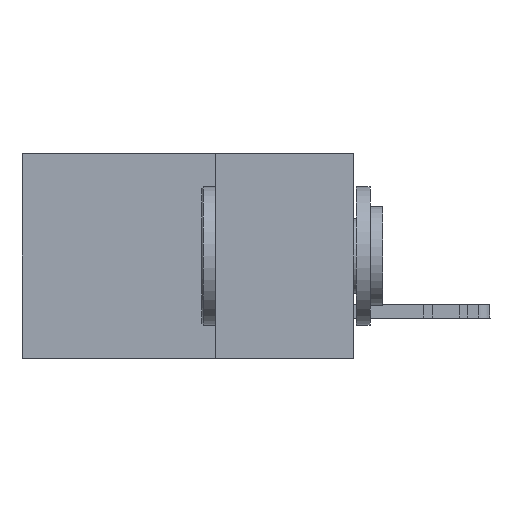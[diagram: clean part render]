
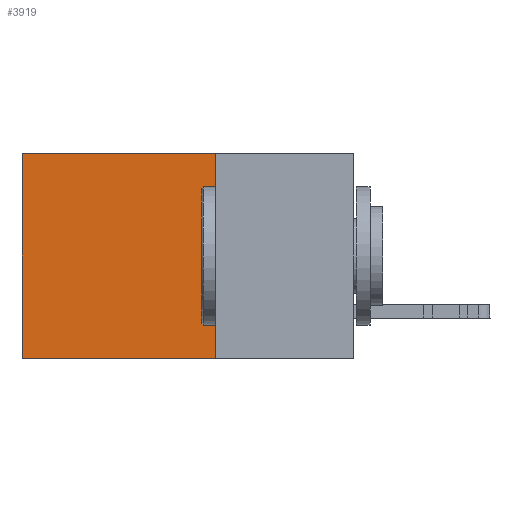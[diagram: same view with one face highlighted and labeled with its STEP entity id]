
A CAD part, left-side view. The second image highlights one B-rep face of the part: STEP entity #3919.
In plain terms, the highlighted planar face has unit normal (-1, 0, 0).
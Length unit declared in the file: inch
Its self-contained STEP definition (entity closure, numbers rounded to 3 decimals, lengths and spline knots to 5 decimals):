
#321 = ORIENTED_EDGE ( 'NONE', *, *, #1398, .T. ) ;
#1398 = EDGE_CURVE ( 'NONE', #1797, #10727, #17160, .T. ) ;
#1447 = CARTESIAN_POINT ( 'NONE',  ( 0.2875, 0.25, -0.37 ) ) ;
#1649 = DIRECTION ( 'NONE',  ( 0., 0., -1. ) ) ;
#1797 = VERTEX_POINT ( 'NONE', #30669 ) ;
#2560 = ORIENTED_EDGE ( 'NONE', *, *, #8829, .F. ) ;
#3861 = ORIENTED_EDGE ( 'NONE', *, *, #10779, .F. ) ;
#3862 = EDGE_LOOP ( 'NONE', ( #321, #3861, #2560, #13032 ) ) ;
#3919 = ADVANCED_FACE ( 'NONE', ( #6775 ), #5761, .F. ) ;
#4377 = DIRECTION ( 'NONE',  ( 0., 1., 0. ) ) ;
#5265 = VECTOR ( 'NONE', #19849, 39.37008 ) ;
#5591 = CARTESIAN_POINT ( 'NONE',  ( 0.2875, 0.6, 0. ) ) ;
#5761 = PLANE ( 'NONE',  #10098 ) ;
#6775 = FACE_OUTER_BOUND ( 'NONE', #3862, .T. ) ;
#7103 = VERTEX_POINT ( 'NONE', #1447 ) ;
#8610 = VECTOR ( 'NONE', #20277, 39.37008 ) ;
#8829 = EDGE_CURVE ( 'NONE', #43433, #7103, #22990, .T. ) ;
#9419 = CARTESIAN_POINT ( 'NONE',  ( 0.2875, 0.25, 0. ) ) ;
#10098 = AXIS2_PLACEMENT_3D ( 'NONE', #9419, #37639, #35231 ) ;
#10727 = VERTEX_POINT ( 'NONE', #28188 ) ;
#10779 = EDGE_CURVE ( 'NONE', #7103, #10727, #31284, .T. ) ;
#13032 = ORIENTED_EDGE ( 'NONE', *, *, #37683, .T. ) ;
#13621 = CARTESIAN_POINT ( 'NONE',  ( 0.2875, 0.25, -0.37 ) ) ;
#17160 = LINE ( 'NONE', #5591, #5265 ) ;
#19849 = DIRECTION ( 'NONE',  ( 0., 0., -1. ) ) ;
#20277 = DIRECTION ( 'NONE',  ( 0., 1., 0. ) ) ;
#22990 = LINE ( 'NONE', #34289, #29772 ) ;
#28188 = CARTESIAN_POINT ( 'NONE',  ( 0.2875, 0.6, -0.37 ) ) ;
#29772 = VECTOR ( 'NONE', #1649, 39.37008 ) ;
#30669 = CARTESIAN_POINT ( 'NONE',  ( 0.2875, 0.6, 0. ) ) ;
#31284 = LINE ( 'NONE', #13621, #8610 ) ;
#32532 = VECTOR ( 'NONE', #4377, 39.37008 ) ;
#33685 = LINE ( 'NONE', #44633, #32532 ) ;
#34289 = CARTESIAN_POINT ( 'NONE',  ( 0.2875, 0.25, 0. ) ) ;
#35231 = DIRECTION ( 'NONE',  ( 0., 0., -1. ) ) ;
#37639 = DIRECTION ( 'NONE',  ( 1., 0., 0. ) ) ;
#37683 = EDGE_CURVE ( 'NONE', #43433, #1797, #33685, .T. ) ;
#41887 = CARTESIAN_POINT ( 'NONE',  ( 0.2875, 0.25, 0. ) ) ;
#43433 = VERTEX_POINT ( 'NONE', #41887 ) ;
#44633 = CARTESIAN_POINT ( 'NONE',  ( 0.2875, 0.25, 0. ) ) ;
